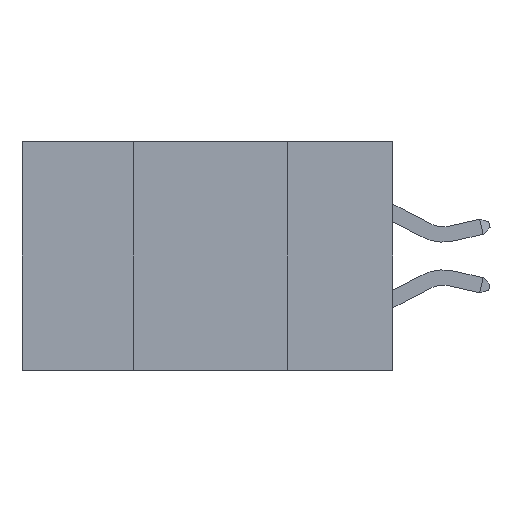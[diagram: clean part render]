
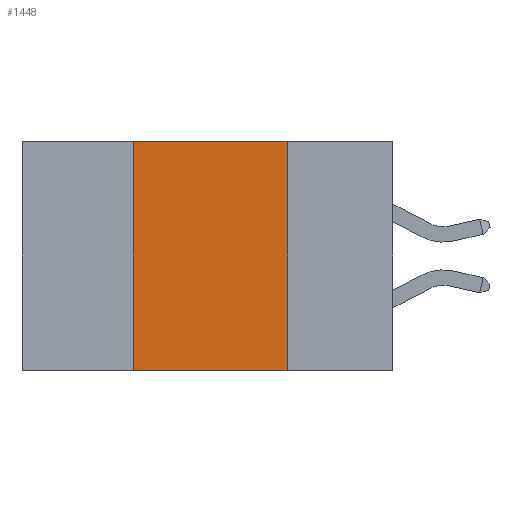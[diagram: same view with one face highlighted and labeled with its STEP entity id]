
A CAD part, left-side view. The second image highlights one B-rep face of the part: STEP entity #1448.
In plain terms, the highlighted planar face has unit normal (-1, 0, 0).
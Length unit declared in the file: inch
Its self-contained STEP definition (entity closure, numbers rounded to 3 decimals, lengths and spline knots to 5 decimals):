
#140 = VERTEX_POINT ( 'NONE', #17225 ) ;
#931 = VECTOR ( 'NONE', #15144, 39.37008 ) ;
#1308 = DIRECTION ( 'NONE',  ( 0., 0., -1. ) ) ;
#1448 = ADVANCED_FACE ( 'NONE', ( #12087 ), #10574, .F. ) ;
#1553 = LINE ( 'NONE', #1640, #9915 ) ;
#1640 = CARTESIAN_POINT ( 'NONE',  ( 0., 0.42, 0. ) ) ;
#1867 = VECTOR ( 'NONE', #11935, 39.37008 ) ;
#2387 = LINE ( 'NONE', #10509, #1867 ) ;
#2440 = ORIENTED_EDGE ( 'NONE', *, *, #3247, .F. ) ;
#2458 = ORIENTED_EDGE ( 'NONE', *, *, #14892, .T. ) ;
#2865 = VERTEX_POINT ( 'NONE', #3138 ) ;
#3138 = CARTESIAN_POINT ( 'NONE',  ( 0., 0.42, 0. ) ) ;
#3247 = EDGE_CURVE ( 'NONE', #12741, #2865, #1553, .T. ) ;
#3661 = CARTESIAN_POINT ( 'NONE',  ( 0., 0.6, 0. ) ) ;
#4074 = LINE ( 'NONE', #4245, #931 ) ;
#4245 = CARTESIAN_POINT ( 'NONE',  ( 0., 0.6, 0. ) ) ;
#4353 = DIRECTION ( 'NONE',  ( 0., 0., 1. ) ) ;
#6499 = EDGE_LOOP ( 'NONE', ( #12540, #13315, #2440, #2458 ) ) ;
#7260 = EDGE_CURVE ( 'NONE', #2865, #15849, #4074, .T. ) ;
#8494 = AXIS2_PLACEMENT_3D ( 'NONE', #3661, #9054, #1308 ) ;
#8816 = CARTESIAN_POINT ( 'NONE',  ( 0., 0.6, -0.37 ) ) ;
#9054 = DIRECTION ( 'NONE',  ( 1., 0., 0. ) ) ;
#9915 = VECTOR ( 'NONE', #4353, 39.37008 ) ;
#10307 = VECTOR ( 'NONE', #16636, 39.37008 ) ;
#10509 = CARTESIAN_POINT ( 'NONE',  ( 0., 0.17, 0. ) ) ;
#10574 = PLANE ( 'NONE',  #8494 ) ;
#11935 = DIRECTION ( 'NONE',  ( 0., 0., -1. ) ) ;
#12087 = FACE_OUTER_BOUND ( 'NONE', #6499, .T. ) ;
#12540 = ORIENTED_EDGE ( 'NONE', *, *, #16572, .F. ) ;
#12741 = VERTEX_POINT ( 'NONE', #14190 ) ;
#13315 = ORIENTED_EDGE ( 'NONE', *, *, #7260, .F. ) ;
#13801 = LINE ( 'NONE', #8816, #10307 ) ;
#14190 = CARTESIAN_POINT ( 'NONE',  ( 0., 0.42, -0.37 ) ) ;
#14193 = CARTESIAN_POINT ( 'NONE',  ( 0., 0.17, 0. ) ) ;
#14892 = EDGE_CURVE ( 'NONE', #12741, #140, #13801, .T. ) ;
#15144 = DIRECTION ( 'NONE',  ( 0., -1., 0. ) ) ;
#15849 = VERTEX_POINT ( 'NONE', #14193 ) ;
#16572 = EDGE_CURVE ( 'NONE', #15849, #140, #2387, .T. ) ;
#16636 = DIRECTION ( 'NONE',  ( 0., -1., 0. ) ) ;
#17225 = CARTESIAN_POINT ( 'NONE',  ( 0., 0.17, -0.37 ) ) ;
